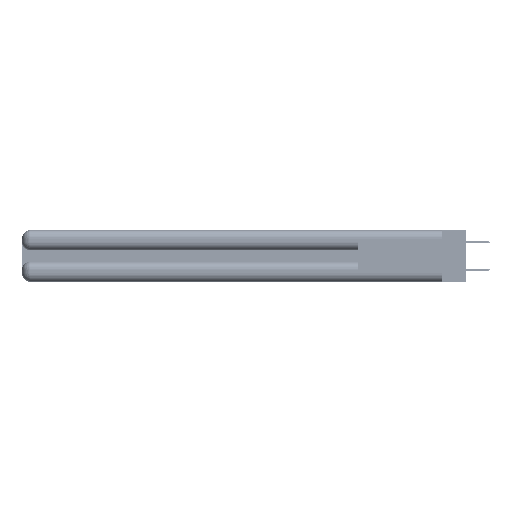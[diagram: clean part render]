
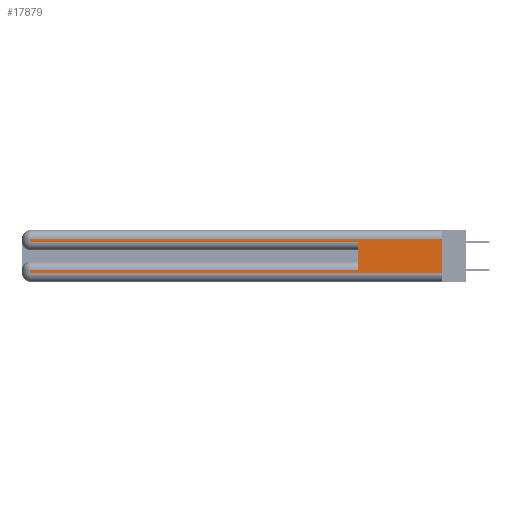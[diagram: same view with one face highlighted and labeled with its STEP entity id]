
A CAD part, left-side view. The second image highlights one B-rep face of the part: STEP entity #17879.
In plain terms, the highlighted planar face has unit normal (-1, 0, 0).
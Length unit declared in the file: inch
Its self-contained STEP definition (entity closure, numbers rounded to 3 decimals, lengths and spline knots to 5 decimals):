
#53 = DIRECTION ( 'NONE',  ( 0., 0., -1. ) ) ;
#312 = CARTESIAN_POINT ( 'NONE',  ( 0., 0., 0.31 ) ) ;
#731 = CARTESIAN_POINT ( 'NONE',  ( 0., 0., 0.37 ) ) ;
#739 = DIRECTION ( 'NONE',  ( 0., 0., -1. ) ) ;
#2446 = ORIENTED_EDGE ( 'NONE', *, *, #31553, .F. ) ;
#2604 = DIRECTION ( 'NONE',  ( 1., 0., 0. ) ) ;
#2667 = LINE ( 'NONE', #30658, #17170 ) ;
#3964 = LINE ( 'NONE', #49838, #10005 ) ;
#5103 = CARTESIAN_POINT ( 'NONE',  ( 0., 2.94, 0.085 ) ) ;
#6165 = ORIENTED_EDGE ( 'NONE', *, *, #19132, .T. ) ;
#6172 = VERTEX_POINT ( 'NONE', #18157 ) ;
#6498 = VECTOR ( 'NONE', #17144, 39.37008 ) ;
#6728 = CARTESIAN_POINT ( 'NONE',  ( 0., 0., 0.31 ) ) ;
#7292 = LINE ( 'NONE', #25344, #24238 ) ;
#8295 = VECTOR ( 'NONE', #46546, 39.37008 ) ;
#8473 = LINE ( 'NONE', #43057, #42330 ) ;
#9014 = EDGE_CURVE ( 'NONE', #15295, #18624, #44789, .T. ) ;
#10005 = VECTOR ( 'NONE', #42241, 39.37008 ) ;
#13298 = CARTESIAN_POINT ( 'NONE',  ( 0., 0., 0.06 ) ) ;
#15112 = CARTESIAN_POINT ( 'NONE',  ( 0., 0., 0.085 ) ) ;
#15295 = VERTEX_POINT ( 'NONE', #6728 ) ;
#15570 = LINE ( 'NONE', #15112, #8295 ) ;
#15694 = FACE_OUTER_BOUND ( 'NONE', #40774, .T. ) ;
#17144 = DIRECTION ( 'NONE',  ( 0., -1., 0. ) ) ;
#17170 = VECTOR ( 'NONE', #53, 39.37008 ) ;
#17344 = LINE ( 'NONE', #47931, #6498 ) ;
#17541 = VERTEX_POINT ( 'NONE', #31324 ) ;
#17879 = ADVANCED_FACE ( 'NONE', ( #15694 ), #33709, .F. ) ;
#18086 = VERTEX_POINT ( 'NONE', #39052 ) ;
#18157 = CARTESIAN_POINT ( 'NONE',  ( 0., 2.94, 0.285 ) ) ;
#18575 = ORIENTED_EDGE ( 'NONE', *, *, #20714, .T. ) ;
#18624 = VERTEX_POINT ( 'NONE', #13298 ) ;
#19132 = EDGE_CURVE ( 'NONE', #48677, #18624, #17344, .T. ) ;
#20133 = DIRECTION ( 'NONE',  ( 0., 1., 0. ) ) ;
#20714 = EDGE_CURVE ( 'NONE', #33281, #48677, #2667, .T. ) ;
#21470 = VERTEX_POINT ( 'NONE', #21870 ) ;
#21870 = CARTESIAN_POINT ( 'NONE',  ( 0., 2.94, 0.31 ) ) ;
#22995 = ORIENTED_EDGE ( 'NONE', *, *, #24198, .T. ) ;
#23533 = ORIENTED_EDGE ( 'NONE', *, *, #49142, .T. ) ;
#24198 = EDGE_CURVE ( 'NONE', #17541, #33281, #15570, .T. ) ;
#24238 = VECTOR ( 'NONE', #32602, 39.37008 ) ;
#25344 = CARTESIAN_POINT ( 'NONE',  ( 0., 0., 0.285 ) ) ;
#26116 = CARTESIAN_POINT ( 'NONE',  ( 0., 0., 0.37 ) ) ;
#29658 = DIRECTION ( 'NONE',  ( 0., 0., -1. ) ) ;
#30658 = CARTESIAN_POINT ( 'NONE',  ( 0., 2.94, 0.37 ) ) ;
#31324 = CARTESIAN_POINT ( 'NONE',  ( 0., 0.6, 0.085 ) ) ;
#31553 = EDGE_CURVE ( 'NONE', #17541, #18086, #3964, .T. ) ;
#32523 = LINE ( 'NONE', #312, #35554 ) ;
#32602 = DIRECTION ( 'NONE',  ( 0., -1., 0. ) ) ;
#33281 = VERTEX_POINT ( 'NONE', #5103 ) ;
#33709 = PLANE ( 'NONE',  #38235 ) ;
#35554 = VECTOR ( 'NONE', #20133, 39.37008 ) ;
#35718 = CARTESIAN_POINT ( 'NONE',  ( 0., 2.94, 0.06 ) ) ;
#36831 = EDGE_CURVE ( 'NONE', #6172, #18086, #7292, .T. ) ;
#36937 = ORIENTED_EDGE ( 'NONE', *, *, #9014, .F. ) ;
#38115 = VECTOR ( 'NONE', #39803, 39.37008 ) ;
#38235 = AXIS2_PLACEMENT_3D ( 'NONE', #26116, #2604, #29658 ) ;
#38801 = ORIENTED_EDGE ( 'NONE', *, *, #41152, .T. ) ;
#39052 = CARTESIAN_POINT ( 'NONE',  ( 0., 0.6, 0.285 ) ) ;
#39803 = DIRECTION ( 'NONE',  ( 0., 0., -1. ) ) ;
#40774 = EDGE_LOOP ( 'NONE', ( #36937, #38801, #23533, #42460, #2446, #22995, #18575, #6165 ) ) ;
#41152 = EDGE_CURVE ( 'NONE', #15295, #21470, #32523, .T. ) ;
#42241 = DIRECTION ( 'NONE',  ( 0., 0., 1. ) ) ;
#42330 = VECTOR ( 'NONE', #739, 39.37008 ) ;
#42460 = ORIENTED_EDGE ( 'NONE', *, *, #36831, .T. ) ;
#43057 = CARTESIAN_POINT ( 'NONE',  ( 0., 2.94, 0.37 ) ) ;
#44789 = LINE ( 'NONE', #731, #38115 ) ;
#46546 = DIRECTION ( 'NONE',  ( 0., 1., 0. ) ) ;
#47931 = CARTESIAN_POINT ( 'NONE',  ( 0., 0., 0.06 ) ) ;
#48677 = VERTEX_POINT ( 'NONE', #35718 ) ;
#49142 = EDGE_CURVE ( 'NONE', #21470, #6172, #8473, .T. ) ;
#49838 = CARTESIAN_POINT ( 'NONE',  ( 0., 0.6, 0.145 ) ) ;
